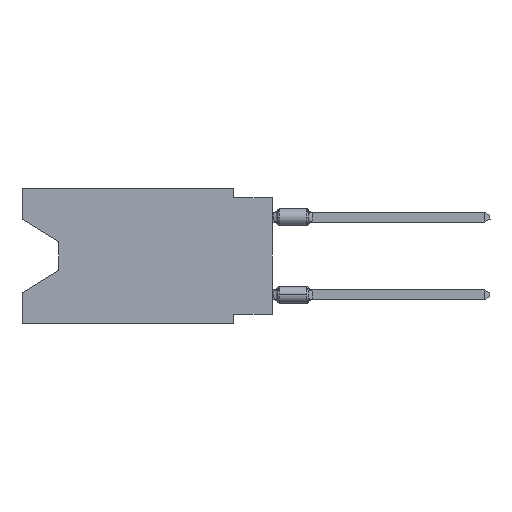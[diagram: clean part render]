
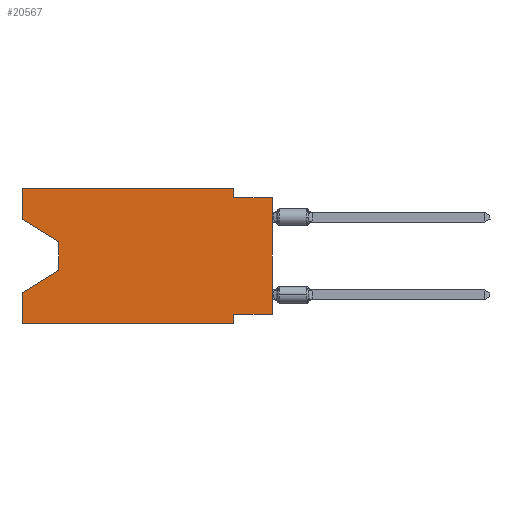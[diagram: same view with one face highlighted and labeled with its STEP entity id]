
A CAD part, left-side view. The second image highlights one B-rep face of the part: STEP entity #20567.
In plain terms, the highlighted planar face has unit normal (-1, 0, 0).
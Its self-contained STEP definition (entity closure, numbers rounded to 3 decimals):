
#3 = VERTEX_POINT ( 'NONE', #36317 ) ;
#427 = AXIS2_PLACEMENT_3D ( 'NONE', #12104, #16216, #8268 ) ;
#573 = VERTEX_POINT ( 'NONE', #28739 ) ;
#896 = DIRECTION ( 'NONE',  ( 0., -1., 0. ) ) ;
#1058 = FACE_OUTER_BOUND ( 'NONE', #25720, .T. ) ;
#1856 = CARTESIAN_POINT ( 'NONE',  ( 0., 16.383, -2.038 ) ) ;
#2078 = EDGE_CURVE ( 'NONE', #23829, #23531, #11007, .T. ) ;
#2292 = CARTESIAN_POINT ( 'NONE',  ( 0., 2.54, -0.635 ) ) ;
#2821 = CARTESIAN_POINT ( 'NONE',  ( 0., 0., -0.635 ) ) ;
#3998 = ORIENTED_EDGE ( 'NONE', *, *, #22447, .F. ) ;
#4135 = LINE ( 'NONE', #15677, #31984 ) ;
#4141 = ORIENTED_EDGE ( 'NONE', *, *, #24902, .T. ) ;
#4510 = CARTESIAN_POINT ( 'NONE',  ( 0., 13.97, -3.505 ) ) ;
#5441 = CARTESIAN_POINT ( 'NONE',  ( 0., 16.383, -6.852 ) ) ;
#6284 = CARTESIAN_POINT ( 'NONE',  ( 0., 13.97, -5.385 ) ) ;
#6802 = LINE ( 'NONE', #10640, #18894 ) ;
#7051 = CARTESIAN_POINT ( 'NONE',  ( 0., 16.383, 0. ) ) ;
#7062 = EDGE_CURVE ( 'NONE', #16850, #43817, #4135, .T. ) ;
#7975 = EDGE_CURVE ( 'NONE', #10124, #3, #26798, .T. ) ;
#8268 = DIRECTION ( 'NONE',  ( 0., 0., -1. ) ) ;
#8531 = CARTESIAN_POINT ( 'NONE',  ( 0., 16.383, 0. ) ) ;
#8672 = ORIENTED_EDGE ( 'NONE', *, *, #10063, .T. ) ;
#9036 = VECTOR ( 'NONE', #45324, 1000. ) ;
#9270 = VECTOR ( 'NONE', #896, 1000. ) ;
#9320 = CARTESIAN_POINT ( 'NONE',  ( 0., 16.383, -2.038 ) ) ;
#9572 = DIRECTION ( 'NONE',  ( 0., -1., 0. ) ) ;
#9597 = VECTOR ( 'NONE', #17043, 1000. ) ;
#9876 = CARTESIAN_POINT ( 'NONE',  ( 0., 0., -8.255 ) ) ;
#10051 = LINE ( 'NONE', #2821, #19646 ) ;
#10063 = EDGE_CURVE ( 'NONE', #10124, #16850, #19913, .T. ) ;
#10124 = VERTEX_POINT ( 'NONE', #1856 ) ;
#10614 = CARTESIAN_POINT ( 'NONE',  ( 0., 13.97, -5.385 ) ) ;
#10640 = CARTESIAN_POINT ( 'NONE',  ( 0., 2.54, -8.89 ) ) ;
#10656 = DIRECTION ( 'NONE',  ( 0., -1., 0. ) ) ;
#10864 = VERTEX_POINT ( 'NONE', #37799 ) ;
#10952 = VECTOR ( 'NONE', #10656, 1000. ) ;
#11007 = LINE ( 'NONE', #41531, #9270 ) ;
#11978 = CARTESIAN_POINT ( 'NONE',  ( 0., 2.54, -8.89 ) ) ;
#12036 = VERTEX_POINT ( 'NONE', #41917 ) ;
#12104 = CARTESIAN_POINT ( 'NONE',  ( 0., 16.383, 0. ) ) ;
#12535 = DIRECTION ( 'NONE',  ( 0., 0., -1. ) ) ;
#13238 = VECTOR ( 'NONE', #42521, 1000. ) ;
#13727 = LINE ( 'NONE', #6284, #32061 ) ;
#14219 = ORIENTED_EDGE ( 'NONE', *, *, #7975, .F. ) ;
#15677 = CARTESIAN_POINT ( 'NONE',  ( 0., 13.97, -3.505 ) ) ;
#16216 = DIRECTION ( 'NONE',  ( 1., 0., 0. ) ) ;
#16261 = ORIENTED_EDGE ( 'NONE', *, *, #45509, .F. ) ;
#16451 = ORIENTED_EDGE ( 'NONE', *, *, #28223, .F. ) ;
#16850 = VERTEX_POINT ( 'NONE', #4510 ) ;
#17043 = DIRECTION ( 'NONE',  ( 0., 0., 1. ) ) ;
#17270 = CARTESIAN_POINT ( 'NONE',  ( 0., 0., 0. ) ) ;
#18894 = VECTOR ( 'NONE', #39977, 1000. ) ;
#18970 = CARTESIAN_POINT ( 'NONE',  ( 0., 0., -8.255 ) ) ;
#18991 = VERTEX_POINT ( 'NONE', #5441 ) ;
#19646 = VECTOR ( 'NONE', #9572, 1000. ) ;
#19913 = LINE ( 'NONE', #9320, #24506 ) ;
#20182 = CARTESIAN_POINT ( 'NONE',  ( 0., 2.54, 0. ) ) ;
#20567 = ADVANCED_FACE ( 'NONE', ( #1058 ), #41459, .F. ) ;
#20842 = EDGE_CURVE ( 'NONE', #573, #23531, #6802, .T. ) ;
#21266 = VECTOR ( 'NONE', #22136, 1000. ) ;
#21976 = CARTESIAN_POINT ( 'NONE',  ( 0., 16.383, 0. ) ) ;
#22062 = EDGE_CURVE ( 'NONE', #23829, #18991, #32524, .T. ) ;
#22086 = CARTESIAN_POINT ( 'NONE',  ( 0., 16.383, -8.89 ) ) ;
#22136 = DIRECTION ( 'NONE',  ( 0., 1., 0. ) ) ;
#22447 = EDGE_CURVE ( 'NONE', #12036, #37272, #38646, .T. ) ;
#23531 = VERTEX_POINT ( 'NONE', #11978 ) ;
#23829 = VERTEX_POINT ( 'NONE', #22086 ) ;
#24421 = VERTEX_POINT ( 'NONE', #9876 ) ;
#24506 = VECTOR ( 'NONE', #45395, 1000. ) ;
#24902 = EDGE_CURVE ( 'NONE', #24421, #10864, #46614, .T. ) ;
#25720 = EDGE_LOOP ( 'NONE', ( #8672, #40587, #28478, #38796, #32486, #31533, #16261, #4141, #16451, #3998, #30848, #14219 ) ) ;
#26798 = LINE ( 'NONE', #8531, #9036 ) ;
#28223 = EDGE_CURVE ( 'NONE', #37272, #10864, #10051, .T. ) ;
#28478 = ORIENTED_EDGE ( 'NONE', *, *, #30218, .T. ) ;
#28739 = CARTESIAN_POINT ( 'NONE',  ( 0., 2.54, -8.255 ) ) ;
#30218 = EDGE_CURVE ( 'NONE', #43817, #18991, #13727, .T. ) ;
#30848 = ORIENTED_EDGE ( 'NONE', *, *, #38230, .F. ) ;
#31533 = ORIENTED_EDGE ( 'NONE', *, *, #20842, .F. ) ;
#31984 = VECTOR ( 'NONE', #12535, 1000. ) ;
#32061 = VECTOR ( 'NONE', #47148, 1000. ) ;
#32293 = DIRECTION ( 'NONE',  ( 0., 0., 1. ) ) ;
#32486 = ORIENTED_EDGE ( 'NONE', *, *, #2078, .T. ) ;
#32524 = LINE ( 'NONE', #7051, #44720 ) ;
#36317 = CARTESIAN_POINT ( 'NONE',  ( 0., 16.383, 0. ) ) ;
#37272 = VERTEX_POINT ( 'NONE', #2292 ) ;
#37799 = CARTESIAN_POINT ( 'NONE',  ( 0., 0., -0.635 ) ) ;
#38230 = EDGE_CURVE ( 'NONE', #3, #12036, #43851, .T. ) ;
#38646 = LINE ( 'NONE', #20182, #13238 ) ;
#38796 = ORIENTED_EDGE ( 'NONE', *, *, #22062, .F. ) ;
#39977 = DIRECTION ( 'NONE',  ( 0., 0., -1. ) ) ;
#40587 = ORIENTED_EDGE ( 'NONE', *, *, #7062, .T. ) ;
#41459 = PLANE ( 'NONE',  #427 ) ;
#41531 = CARTESIAN_POINT ( 'NONE',  ( 0., 16.383, -8.89 ) ) ;
#41917 = CARTESIAN_POINT ( 'NONE',  ( 0., 2.54, 0. ) ) ;
#42521 = DIRECTION ( 'NONE',  ( 0., 0., -1. ) ) ;
#43817 = VERTEX_POINT ( 'NONE', #10614 ) ;
#43851 = LINE ( 'NONE', #21976, #10952 ) ;
#44466 = LINE ( 'NONE', #18970, #21266 ) ;
#44720 = VECTOR ( 'NONE', #32293, 1000. ) ;
#45324 = DIRECTION ( 'NONE',  ( 0., 0., 1. ) ) ;
#45395 = DIRECTION ( 'NONE',  ( 0., -0.855, -0.519 ) ) ;
#45509 = EDGE_CURVE ( 'NONE', #24421, #573, #44466, .T. ) ;
#46614 = LINE ( 'NONE', #17270, #9597 ) ;
#47148 = DIRECTION ( 'NONE',  ( 0., 0.855, -0.519 ) ) ;
